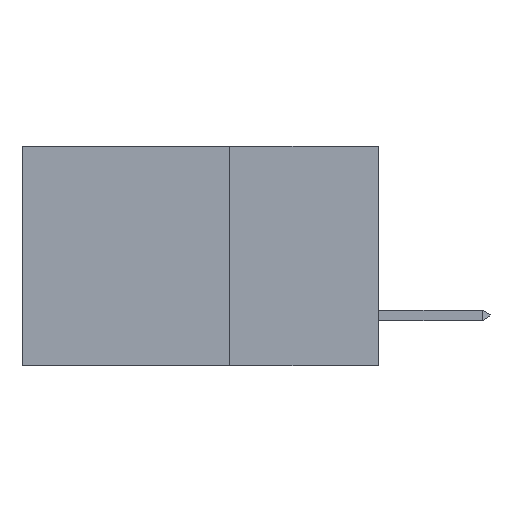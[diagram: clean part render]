
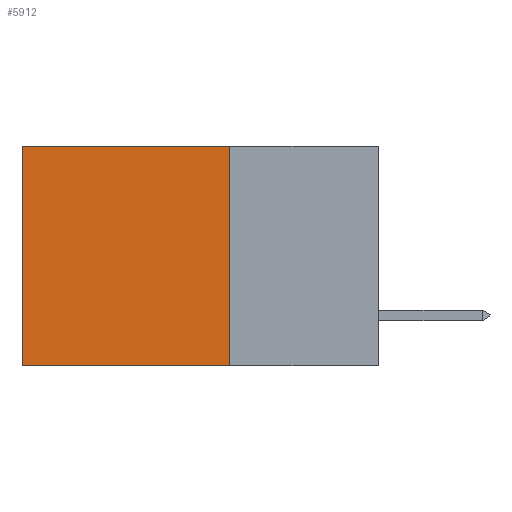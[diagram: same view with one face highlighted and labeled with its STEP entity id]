
A CAD part, left-side view. The second image highlights one B-rep face of the part: STEP entity #5912.
In plain terms, the highlighted planar face has unit normal (-1, 0, 0).
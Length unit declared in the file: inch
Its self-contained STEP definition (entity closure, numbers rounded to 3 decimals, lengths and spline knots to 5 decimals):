
#269 = PLANE ( 'NONE',  #7132 ) ;
#512 = LINE ( 'NONE', #9145, #5508 ) ;
#892 = ORIENTED_EDGE ( 'NONE', *, *, #10735, .T. ) ;
#1145 = EDGE_CURVE ( 'NONE', #6116, #9716, #7068, .T. ) ;
#1188 = DIRECTION ( 'NONE',  ( 0., 1., 0. ) ) ;
#1724 = DIRECTION ( 'NONE',  ( 0., 0., -1. ) ) ;
#1827 = LINE ( 'NONE', #6986, #4963 ) ;
#2053 = CARTESIAN_POINT ( 'NONE',  ( 0.2615, 0.25, -0.37 ) ) ;
#2745 = FACE_OUTER_BOUND ( 'NONE', #10189, .T. ) ;
#2868 = ORIENTED_EDGE ( 'NONE', *, *, #6177, .F. ) ;
#3477 = VERTEX_POINT ( 'NONE', #8860 ) ;
#4087 = CARTESIAN_POINT ( 'NONE',  ( 0.2615, 0.25, -0.37 ) ) ;
#4890 = LINE ( 'NONE', #4087, #7360 ) ;
#4963 = VECTOR ( 'NONE', #5181, 39.37008 ) ;
#5130 = ORIENTED_EDGE ( 'NONE', *, *, #1145, .T. ) ;
#5181 = DIRECTION ( 'NONE',  ( 0., 0., -1. ) ) ;
#5508 = VECTOR ( 'NONE', #7233, 39.37008 ) ;
#5912 = ADVANCED_FACE ( 'NONE', ( #2745 ), #269, .F. ) ;
#6116 = VERTEX_POINT ( 'NONE', #8913 ) ;
#6177 = EDGE_CURVE ( 'NONE', #9961, #3477, #4890, .T. ) ;
#6924 = CARTESIAN_POINT ( 'NONE',  ( 0.2615, 0.25, -0.37 ) ) ;
#6986 = CARTESIAN_POINT ( 'NONE',  ( 0.2615, 0.25, -0.37 ) ) ;
#7068 = LINE ( 'NONE', #8835, #9336 ) ;
#7132 = AXIS2_PLACEMENT_3D ( 'NONE', #6924, #7870, #1724 ) ;
#7233 = DIRECTION ( 'NONE',  ( 0., 0., -1. ) ) ;
#7360 = VECTOR ( 'NONE', #9125, 39.37008 ) ;
#7870 = DIRECTION ( 'NONE',  ( 1., 0., 0. ) ) ;
#8388 = CARTESIAN_POINT ( 'NONE',  ( 0.2615, 0.6, 0. ) ) ;
#8835 = CARTESIAN_POINT ( 'NONE',  ( 0.2615, 0.25, 0. ) ) ;
#8860 = CARTESIAN_POINT ( 'NONE',  ( 0.2615, 0.6, -0.37 ) ) ;
#8913 = CARTESIAN_POINT ( 'NONE',  ( 0.2615, 0.25, 0. ) ) ;
#9125 = DIRECTION ( 'NONE',  ( 0., 1., 0. ) ) ;
#9145 = CARTESIAN_POINT ( 'NONE',  ( 0.2615, 0.6, -0.37 ) ) ;
#9336 = VECTOR ( 'NONE', #1188, 39.37008 ) ;
#9716 = VERTEX_POINT ( 'NONE', #8388 ) ;
#9863 = EDGE_CURVE ( 'NONE', #6116, #9961, #1827, .T. ) ;
#9961 = VERTEX_POINT ( 'NONE', #2053 ) ;
#10189 = EDGE_LOOP ( 'NONE', ( #892, #2868, #10518, #5130 ) ) ;
#10518 = ORIENTED_EDGE ( 'NONE', *, *, #9863, .F. ) ;
#10735 = EDGE_CURVE ( 'NONE', #9716, #3477, #512, .T. ) ;
